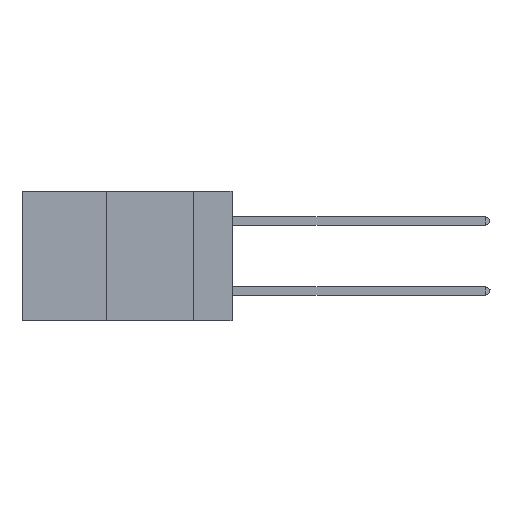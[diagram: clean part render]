
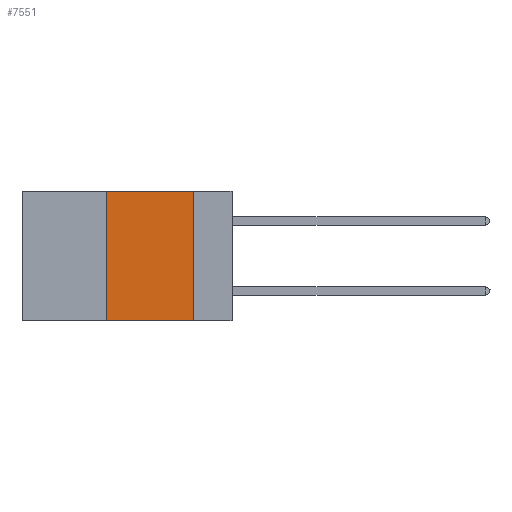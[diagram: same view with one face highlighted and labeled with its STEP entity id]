
A CAD part, left-side view. The second image highlights one B-rep face of the part: STEP entity #7551.
In plain terms, the highlighted planar face has unit normal (-1, 0, 0).
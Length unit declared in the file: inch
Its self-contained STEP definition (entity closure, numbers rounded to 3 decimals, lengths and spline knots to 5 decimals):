
#630 = DIRECTION ( 'NONE',  ( 0., 0., 1. ) ) ;
#978 = VERTEX_POINT ( 'NONE', #13998 ) ;
#1862 = AXIS2_PLACEMENT_3D ( 'NONE', #6553, #22753, #23320 ) ;
#2272 = CARTESIAN_POINT ( 'NONE',  ( 0., 0.11, -0.37 ) ) ;
#3397 = PLANE ( 'NONE',  #1862 ) ;
#4255 = ORIENTED_EDGE ( 'NONE', *, *, #7021, .F. ) ;
#4345 = EDGE_CURVE ( 'NONE', #20919, #6277, #19265, .T. ) ;
#4862 = EDGE_LOOP ( 'NONE', ( #17484, #4255, #10727, #21424 ) ) ;
#6277 = VERTEX_POINT ( 'NONE', #10062 ) ;
#6527 = VECTOR ( 'NONE', #21067, 39.37008 ) ;
#6553 = CARTESIAN_POINT ( 'NONE',  ( 0., 0.6, 0. ) ) ;
#7021 = EDGE_CURVE ( 'NONE', #6277, #978, #21732, .T. ) ;
#7551 = ADVANCED_FACE ( 'NONE', ( #8786 ), #3397, .F. ) ;
#7757 = CARTESIAN_POINT ( 'NONE',  ( 0., 0.36, 0. ) ) ;
#8786 = FACE_OUTER_BOUND ( 'NONE', #4862, .T. ) ;
#9155 = DIRECTION ( 'NONE',  ( 0., 0., -1. ) ) ;
#10062 = CARTESIAN_POINT ( 'NONE',  ( 0., 0.36, 0. ) ) ;
#10689 = CARTESIAN_POINT ( 'NONE',  ( 0., 0.6, 0. ) ) ;
#10727 = ORIENTED_EDGE ( 'NONE', *, *, #4345, .F. ) ;
#11046 = LINE ( 'NONE', #12811, #22024 ) ;
#12811 = CARTESIAN_POINT ( 'NONE',  ( 0., 0.11, 0. ) ) ;
#13417 = DIRECTION ( 'NONE',  ( 0., -1., 0. ) ) ;
#13998 = CARTESIAN_POINT ( 'NONE',  ( 0., 0.11, 0. ) ) ;
#14663 = VECTOR ( 'NONE', #13417, 39.37008 ) ;
#17484 = ORIENTED_EDGE ( 'NONE', *, *, #18888, .F. ) ;
#17584 = VECTOR ( 'NONE', #630, 39.37008 ) ;
#17723 = VERTEX_POINT ( 'NONE', #2272 ) ;
#17777 = LINE ( 'NONE', #23036, #6527 ) ;
#18485 = CARTESIAN_POINT ( 'NONE',  ( 0., 0.36, -0.37 ) ) ;
#18888 = EDGE_CURVE ( 'NONE', #978, #17723, #11046, .T. ) ;
#19260 = EDGE_CURVE ( 'NONE', #20919, #17723, #17777, .T. ) ;
#19265 = LINE ( 'NONE', #7757, #17584 ) ;
#20919 = VERTEX_POINT ( 'NONE', #18485 ) ;
#21067 = DIRECTION ( 'NONE',  ( 0., -1., 0. ) ) ;
#21424 = ORIENTED_EDGE ( 'NONE', *, *, #19260, .T. ) ;
#21732 = LINE ( 'NONE', #10689, #14663 ) ;
#22024 = VECTOR ( 'NONE', #9155, 39.37008 ) ;
#22753 = DIRECTION ( 'NONE',  ( 1., 0., 0. ) ) ;
#23036 = CARTESIAN_POINT ( 'NONE',  ( 0., 0.6, -0.37 ) ) ;
#23320 = DIRECTION ( 'NONE',  ( 0., 0., -1. ) ) ;
